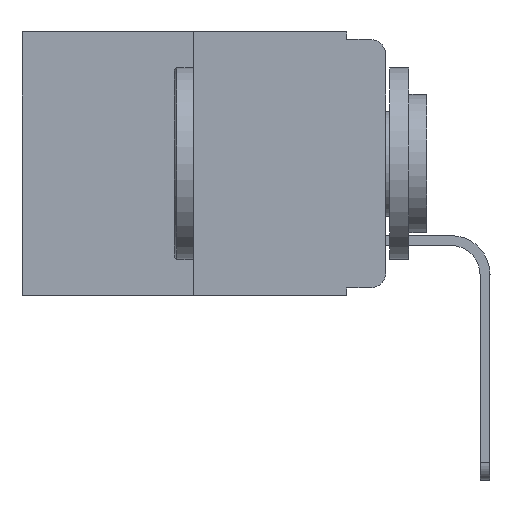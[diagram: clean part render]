
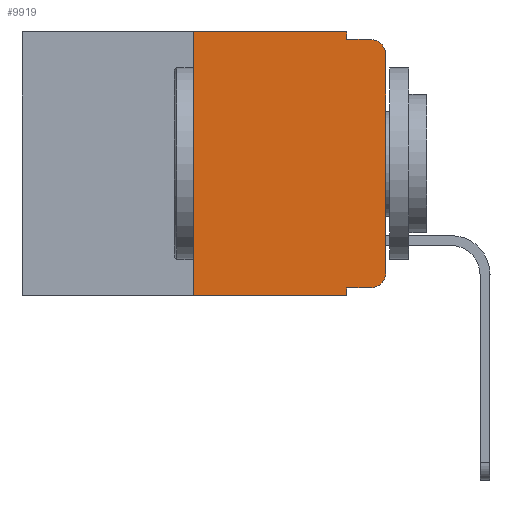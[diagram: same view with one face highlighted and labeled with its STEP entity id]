
A CAD part, left-side view. The second image highlights one B-rep face of the part: STEP entity #9919.
In plain terms, the highlighted planar face has unit normal (-1, 0, 0).
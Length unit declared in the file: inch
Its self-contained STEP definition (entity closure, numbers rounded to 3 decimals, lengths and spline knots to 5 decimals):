
#27 = CARTESIAN_POINT ( 'NONE',  ( 0., 0.02, -0.313 ) ) ;
#39 = CARTESIAN_POINT ( 'NONE',  ( 0., 0.473, 0. ) ) ;
#118 = DIRECTION ( 'NONE',  ( 0., 0., -1. ) ) ;
#241 = CARTESIAN_POINT ( 'NONE',  ( 0., 0., 0. ) ) ;
#350 = FACE_OUTER_BOUND ( 'NONE', #13988, .T. ) ;
#437 = DIRECTION ( 'NONE',  ( 0., -1., 0. ) ) ;
#806 = LINE ( 'NONE', #2575, #9025 ) ;
#960 = EDGE_CURVE ( 'NONE', #10080, #2340, #13783, .T. ) ;
#1254 = VECTOR ( 'NONE', #5722, 39.37008 ) ;
#1293 = VERTEX_POINT ( 'NONE', #4737 ) ;
#1342 = EDGE_CURVE ( 'NONE', #7763, #6678, #7878, .T. ) ;
#1551 = VECTOR ( 'NONE', #118, 39.37008 ) ;
#1609 = ORIENTED_EDGE ( 'NONE', *, *, #1342, .T. ) ;
#1621 = CARTESIAN_POINT ( 'NONE',  ( 0., 0.473, -0.343 ) ) ;
#1846 = CARTESIAN_POINT ( 'NONE',  ( 0., 0.02, -0.333 ) ) ;
#2233 = VECTOR ( 'NONE', #6122, 39.37008 ) ;
#2340 = VERTEX_POINT ( 'NONE', #6635 ) ;
#2387 = CARTESIAN_POINT ( 'NONE',  ( 0., 0.02, -0.03 ) ) ;
#2492 = ORIENTED_EDGE ( 'NONE', *, *, #960, .T. ) ;
#2575 = CARTESIAN_POINT ( 'NONE',  ( 0., 0.051, -0.01 ) ) ;
#2608 = VERTEX_POINT ( 'NONE', #1846 ) ;
#2801 = VERTEX_POINT ( 'NONE', #10998 ) ;
#3155 = EDGE_CURVE ( 'NONE', #4476, #2608, #3641, .T. ) ;
#3271 = EDGE_CURVE ( 'NONE', #2608, #7763, #5022, .T. ) ;
#3359 = ORIENTED_EDGE ( 'NONE', *, *, #13686, .F. ) ;
#3641 = LINE ( 'NONE', #9419, #2233 ) ;
#3772 = LINE ( 'NONE', #13477, #10887 ) ;
#3839 = LINE ( 'NONE', #5703, #1551 ) ;
#4476 = VERTEX_POINT ( 'NONE', #12475 ) ;
#4490 = EDGE_CURVE ( 'NONE', #2801, #1293, #806, .T. ) ;
#4548 = CARTESIAN_POINT ( 'NONE',  ( 0., 0.051, 0. ) ) ;
#4731 = ORIENTED_EDGE ( 'NONE', *, *, #4490, .F. ) ;
#4737 = CARTESIAN_POINT ( 'NONE',  ( 0., 0.02, -0.01 ) ) ;
#4786 = DIRECTION ( 'NONE',  ( 0., 0., 1. ) ) ;
#5022 = CIRCLE ( 'NONE', #9578, 0.02 ) ;
#5313 = CARTESIAN_POINT ( 'NONE',  ( 0., 0.473, 0. ) ) ;
#5409 = DIRECTION ( 'NONE',  ( 0., 0., -1. ) ) ;
#5703 = CARTESIAN_POINT ( 'NONE',  ( 0., 0.051, 0. ) ) ;
#5722 = DIRECTION ( 'NONE',  ( 0., 0., 1. ) ) ;
#6122 = DIRECTION ( 'NONE',  ( 0., -1., 0. ) ) ;
#6130 = ORIENTED_EDGE ( 'NONE', *, *, #6368, .T. ) ;
#6167 = LINE ( 'NONE', #7622, #9997 ) ;
#6368 = EDGE_CURVE ( 'NONE', #6678, #1293, #13158, .T. ) ;
#6381 = CARTESIAN_POINT ( 'NONE',  ( 0., 0., -0.313 ) ) ;
#6427 = DIRECTION ( 'NONE',  ( 1., 0., 0. ) ) ;
#6529 = PLANE ( 'NONE',  #7474 ) ;
#6635 = CARTESIAN_POINT ( 'NONE',  ( 0., 0.051, -0.343 ) ) ;
#6666 = EDGE_CURVE ( 'NONE', #10080, #13998, #3772, .T. ) ;
#6678 = VERTEX_POINT ( 'NONE', #6862 ) ;
#6862 = CARTESIAN_POINT ( 'NONE',  ( 0., 0., -0.03 ) ) ;
#7164 = CARTESIAN_POINT ( 'NONE',  ( 0., 0.25, 0. ) ) ;
#7410 = EDGE_CURVE ( 'NONE', #11869, #2801, #6167, .T. ) ;
#7474 = AXIS2_PLACEMENT_3D ( 'NONE', #5313, #6427, #5409 ) ;
#7622 = CARTESIAN_POINT ( 'NONE',  ( 0., 0.051, 0. ) ) ;
#7763 = VERTEX_POINT ( 'NONE', #6381 ) ;
#7878 = LINE ( 'NONE', #241, #1254 ) ;
#8547 = DIRECTION ( 'NONE',  ( -1., 0., 0. ) ) ;
#9025 = VECTOR ( 'NONE', #12511, 39.37008 ) ;
#9150 = DIRECTION ( 'NONE',  ( 0., 0., -1. ) ) ;
#9419 = CARTESIAN_POINT ( 'NONE',  ( 0., 0.051, -0.333 ) ) ;
#9578 = AXIS2_PLACEMENT_3D ( 'NONE', #27, #8547, #9150 ) ;
#9848 = DIRECTION ( 'NONE',  ( 0., 0., -1. ) ) ;
#9919 = ADVANCED_FACE ( 'NONE', ( #350 ), #6529, .F. ) ;
#9924 = DIRECTION ( 'NONE',  ( 0., -1., 0. ) ) ;
#9979 = CARTESIAN_POINT ( 'NONE',  ( 0., 0.25, -0.343 ) ) ;
#9997 = VECTOR ( 'NONE', #9848, 39.37008 ) ;
#10080 = VERTEX_POINT ( 'NONE', #9979 ) ;
#10108 = ORIENTED_EDGE ( 'NONE', *, *, #3271, .T. ) ;
#10161 = DIRECTION ( 'NONE',  ( -1., 0., 0. ) ) ;
#10547 = VECTOR ( 'NONE', #9924, 39.37008 ) ;
#10887 = VECTOR ( 'NONE', #4786, 39.37008 ) ;
#10998 = CARTESIAN_POINT ( 'NONE',  ( 0., 0.051, -0.01 ) ) ;
#11324 = ORIENTED_EDGE ( 'NONE', *, *, #6666, .F. ) ;
#11459 = DIRECTION ( 'NONE',  ( 0., 0., -1. ) ) ;
#11547 = ORIENTED_EDGE ( 'NONE', *, *, #3155, .T. ) ;
#11680 = ORIENTED_EDGE ( 'NONE', *, *, #11757, .F. ) ;
#11714 = ORIENTED_EDGE ( 'NONE', *, *, #7410, .F. ) ;
#11757 = EDGE_CURVE ( 'NONE', #13998, #11869, #14222, .T. ) ;
#11869 = VERTEX_POINT ( 'NONE', #4548 ) ;
#12475 = CARTESIAN_POINT ( 'NONE',  ( 0., 0.051, -0.333 ) ) ;
#12511 = DIRECTION ( 'NONE',  ( 0., -1., 0. ) ) ;
#12758 = AXIS2_PLACEMENT_3D ( 'NONE', #2387, #10161, #11459 ) ;
#13158 = CIRCLE ( 'NONE', #12758, 0.02 ) ;
#13477 = CARTESIAN_POINT ( 'NONE',  ( 0., 0.25, 0. ) ) ;
#13686 = EDGE_CURVE ( 'NONE', #4476, #2340, #3839, .T. ) ;
#13783 = LINE ( 'NONE', #1621, #13958 ) ;
#13958 = VECTOR ( 'NONE', #437, 39.37008 ) ;
#13988 = EDGE_LOOP ( 'NONE', ( #1609, #6130, #4731, #11714, #11680, #11324, #2492, #3359, #11547, #10108 ) ) ;
#13998 = VERTEX_POINT ( 'NONE', #7164 ) ;
#14222 = LINE ( 'NONE', #39, #10547 ) ;
